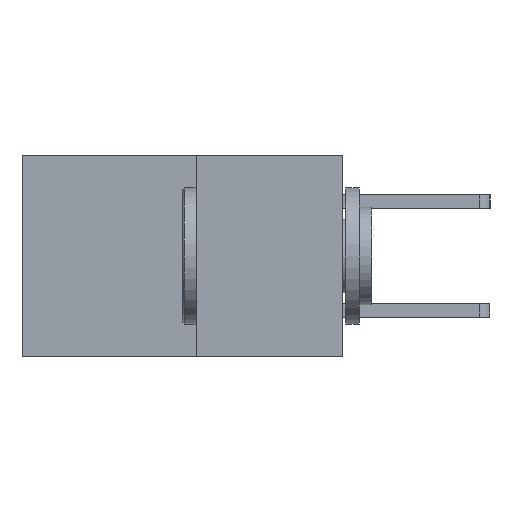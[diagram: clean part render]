
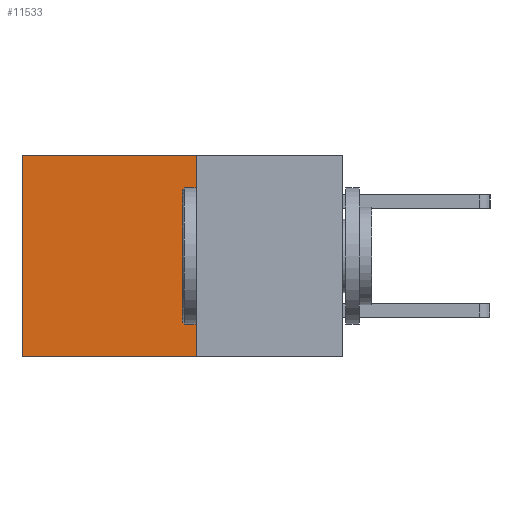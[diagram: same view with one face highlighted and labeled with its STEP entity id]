
A CAD part, left-side view. The second image highlights one B-rep face of the part: STEP entity #11533.
In plain terms, the highlighted planar face has unit normal (-1, 0, 0).
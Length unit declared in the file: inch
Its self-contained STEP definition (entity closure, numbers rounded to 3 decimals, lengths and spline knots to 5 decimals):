
#48 = CARTESIAN_POINT ( 'NONE',  ( 0.277, 0.59, -0.37 ) ) ;
#165 = CARTESIAN_POINT ( 'NONE',  ( 0.277, 0.59, -0.37 ) ) ;
#269 = LINE ( 'NONE', #5398, #2440 ) ;
#513 = CARTESIAN_POINT ( 'NONE',  ( 0.277, 0.27, -0.37 ) ) ;
#657 = DIRECTION ( 'NONE',  ( 0., 1., 0. ) ) ;
#662 = VECTOR ( 'NONE', #2564, 39.37008 ) ;
#800 = CARTESIAN_POINT ( 'NONE',  ( 0.277, 0.27, -0.37 ) ) ;
#1427 = VERTEX_POINT ( 'NONE', #2448 ) ;
#1622 = EDGE_CURVE ( 'NONE', #4229, #11195, #8032, .T. ) ;
#1634 = DIRECTION ( 'NONE',  ( 1., 0., 0. ) ) ;
#1956 = EDGE_CURVE ( 'NONE', #1427, #4229, #4614, .T. ) ;
#2390 = VECTOR ( 'NONE', #6627, 39.37008 ) ;
#2440 = VECTOR ( 'NONE', #657, 39.37008 ) ;
#2448 = CARTESIAN_POINT ( 'NONE',  ( 0.277, 0.27, 0. ) ) ;
#2564 = DIRECTION ( 'NONE',  ( 0., 1., 0. ) ) ;
#3071 = EDGE_CURVE ( 'NONE', #9730, #11195, #10112, .T. ) ;
#3599 = AXIS2_PLACEMENT_3D ( 'NONE', #7417, #1634, #8377 ) ;
#4229 = VERTEX_POINT ( 'NONE', #800 ) ;
#4399 = ORIENTED_EDGE ( 'NONE', *, *, #11512, .T. ) ;
#4614 = LINE ( 'NONE', #4733, #2390 ) ;
#4668 = CARTESIAN_POINT ( 'NONE',  ( 0.277, 0.59, 0. ) ) ;
#4733 = CARTESIAN_POINT ( 'NONE',  ( 0.277, 0.27, -0.37 ) ) ;
#5349 = ORIENTED_EDGE ( 'NONE', *, *, #3071, .T. ) ;
#5398 = CARTESIAN_POINT ( 'NONE',  ( 0.277, 0.27, 0. ) ) ;
#6627 = DIRECTION ( 'NONE',  ( 0., 0., -1. ) ) ;
#6985 = FACE_OUTER_BOUND ( 'NONE', #8487, .T. ) ;
#7417 = CARTESIAN_POINT ( 'NONE',  ( 0.277, 0.27, -0.37 ) ) ;
#8032 = LINE ( 'NONE', #513, #662 ) ;
#8377 = DIRECTION ( 'NONE',  ( 0., 0., -1. ) ) ;
#8487 = EDGE_LOOP ( 'NONE', ( #5349, #10603, #9253, #4399 ) ) ;
#8513 = DIRECTION ( 'NONE',  ( 0., 0., -1. ) ) ;
#9249 = PLANE ( 'NONE',  #3599 ) ;
#9253 = ORIENTED_EDGE ( 'NONE', *, *, #1956, .F. ) ;
#9730 = VERTEX_POINT ( 'NONE', #4668 ) ;
#9828 = VECTOR ( 'NONE', #8513, 39.37008 ) ;
#10112 = LINE ( 'NONE', #48, #9828 ) ;
#10603 = ORIENTED_EDGE ( 'NONE', *, *, #1622, .F. ) ;
#11195 = VERTEX_POINT ( 'NONE', #165 ) ;
#11512 = EDGE_CURVE ( 'NONE', #1427, #9730, #269, .T. ) ;
#11533 = ADVANCED_FACE ( 'NONE', ( #6985 ), #9249, .F. ) ;
